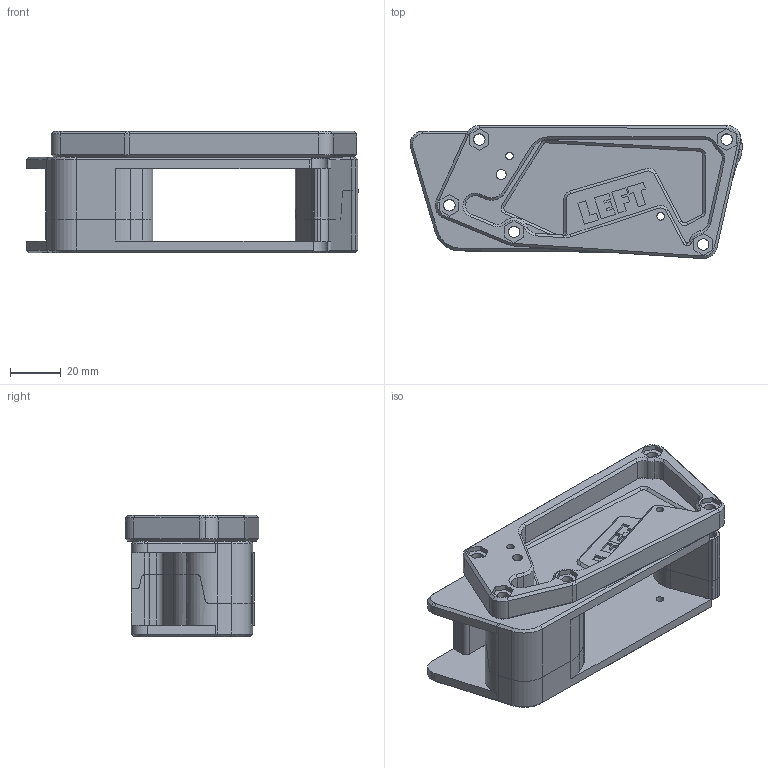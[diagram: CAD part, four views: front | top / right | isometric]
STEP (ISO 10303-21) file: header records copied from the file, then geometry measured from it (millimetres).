
FILE_DESCRIPTION (( 'STEP AP214' ), '1' );
FILE_NAME ('P80G19 JIG MM Kinder Egg.STEP', '2022-09-08T04:06:14', ( '' ), ( '' ), 'SwSTEP 2.0', 'SolidWorks 2020', '' );
FILE_SCHEMA (( 'AUTOMOTIVE_DESIGN' ));
Length unit declared in the file: inch
Products named in the file (3): P80G19 JIG MM Kinder Egg; P8019_Jig_V4_+Guide; Drill Guide^P80G19 JIG MM Remix
Assembly tree (2 placements, depth 2):
  P80G19 JIG MM Kinder Egg
    P8019_Jig_V4_+Guide
    Drill Guide^P80G19 JIG MM Remix
Bounding box: 130.56 x 52.38 x 47.7 mm (x, y, z)
Volume: 113159.9 mm3; surface area: 49370.4 mm2
Topology: 3 solids, 3 shells, 1059 faces, 2887 edges, 1881 vertices
Faces by surface type: plane 545, bspline 206, cylinder 189, cone 119
Entity records: 40796 total; most frequent: CARTESIAN_POINT 13881, ORIENTED_EDGE 5774, DIRECTION 4500, EDGE_CURVE 2887, VERTEX_POINT 1881, LINE 1872, VECTOR 1872, AXIS2_PLACEMENT_3D 1314
